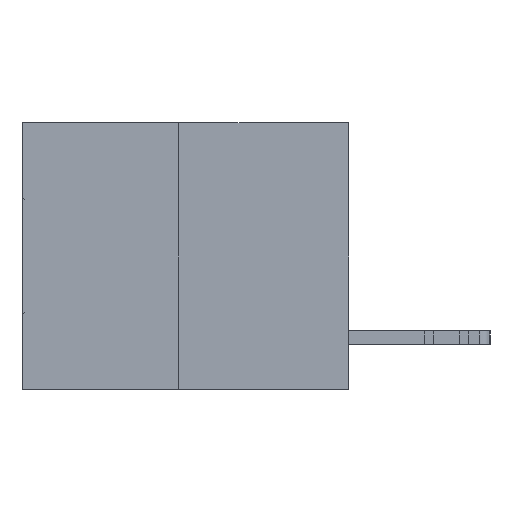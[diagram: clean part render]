
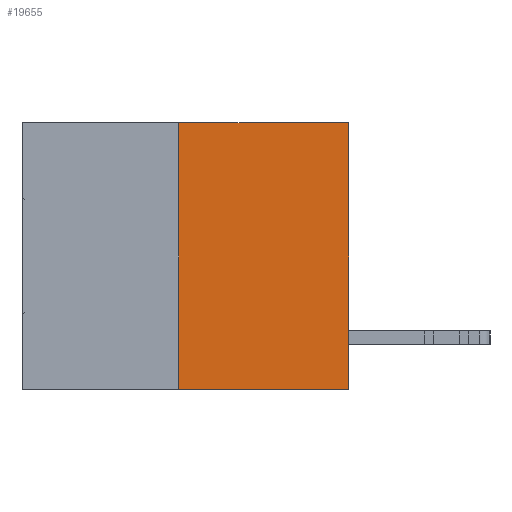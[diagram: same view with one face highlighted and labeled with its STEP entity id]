
A CAD part, left-side view. The second image highlights one B-rep face of the part: STEP entity #19655.
In plain terms, the highlighted planar face has unit normal (-1, 0, 0).
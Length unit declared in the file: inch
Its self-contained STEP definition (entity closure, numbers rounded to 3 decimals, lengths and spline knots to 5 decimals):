
#1896 = CARTESIAN_POINT ( 'NONE',  ( 0., 0.6, 0. ) ) ;
#2032 = AXIS2_PLACEMENT_3D ( 'NONE', #1896, #27243, #28597 ) ;
#4075 = ORIENTED_EDGE ( 'NONE', *, *, #19938, .F. ) ;
#4227 = ORIENTED_EDGE ( 'NONE', *, *, #32519, .T. ) ;
#5698 = VERTEX_POINT ( 'NONE', #6068 ) ;
#6068 = CARTESIAN_POINT ( 'NONE',  ( 0., 0.312, 0. ) ) ;
#6833 = CARTESIAN_POINT ( 'NONE',  ( 0., 0.6, 0. ) ) ;
#7094 = VECTOR ( 'NONE', #10264, 39.37008 ) ;
#9052 = DIRECTION ( 'NONE',  ( 0., 0., 1. ) ) ;
#9218 = LINE ( 'NONE', #32801, #26590 ) ;
#9721 = CARTESIAN_POINT ( 'NONE',  ( 0., 0., 0. ) ) ;
#10264 = DIRECTION ( 'NONE',  ( 0., -1., 0. ) ) ;
#11357 = EDGE_CURVE ( 'NONE', #5698, #28943, #30769, .T. ) ;
#12561 = ORIENTED_EDGE ( 'NONE', *, *, #11357, .F. ) ;
#12594 = VERTEX_POINT ( 'NONE', #31635 ) ;
#13889 = VERTEX_POINT ( 'NONE', #25169 ) ;
#14683 = EDGE_LOOP ( 'NONE', ( #4075, #4227, #23797, #12561 ) ) ;
#14973 = VECTOR ( 'NONE', #30412, 39.37008 ) ;
#17472 = VECTOR ( 'NONE', #26021, 39.37008 ) ;
#19655 = ADVANCED_FACE ( 'NONE', ( #25807 ), #25123, .F. ) ;
#19938 = EDGE_CURVE ( 'NONE', #13889, #5698, #9218, .T. ) ;
#22893 = LINE ( 'NONE', #32769, #7094 ) ;
#23797 = ORIENTED_EDGE ( 'NONE', *, *, #28024, .T. ) ;
#25123 = PLANE ( 'NONE',  #2032 ) ;
#25169 = CARTESIAN_POINT ( 'NONE',  ( 0., 0.312, -0.49 ) ) ;
#25807 = FACE_OUTER_BOUND ( 'NONE', #14683, .T. ) ;
#26021 = DIRECTION ( 'NONE',  ( 0., -1., 0. ) ) ;
#26590 = VECTOR ( 'NONE', #9052, 39.37008 ) ;
#27134 = LINE ( 'NONE', #9721, #14973 ) ;
#27243 = DIRECTION ( 'NONE',  ( 1., 0., 0. ) ) ;
#28024 = EDGE_CURVE ( 'NONE', #12594, #28943, #27134, .T. ) ;
#28485 = CARTESIAN_POINT ( 'NONE',  ( 0., 0., 0. ) ) ;
#28597 = DIRECTION ( 'NONE',  ( 0., 0., -1. ) ) ;
#28943 = VERTEX_POINT ( 'NONE', #28485 ) ;
#30412 = DIRECTION ( 'NONE',  ( 0., 0., 1. ) ) ;
#30769 = LINE ( 'NONE', #6833, #17472 ) ;
#31635 = CARTESIAN_POINT ( 'NONE',  ( 0., 0., -0.49 ) ) ;
#32519 = EDGE_CURVE ( 'NONE', #13889, #12594, #22893, .T. ) ;
#32769 = CARTESIAN_POINT ( 'NONE',  ( 0., 0.6, -0.49 ) ) ;
#32801 = CARTESIAN_POINT ( 'NONE',  ( 0., 0.312, -0.49 ) ) ;
